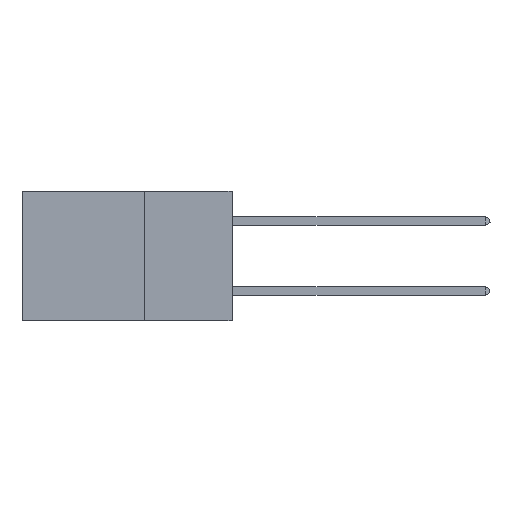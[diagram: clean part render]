
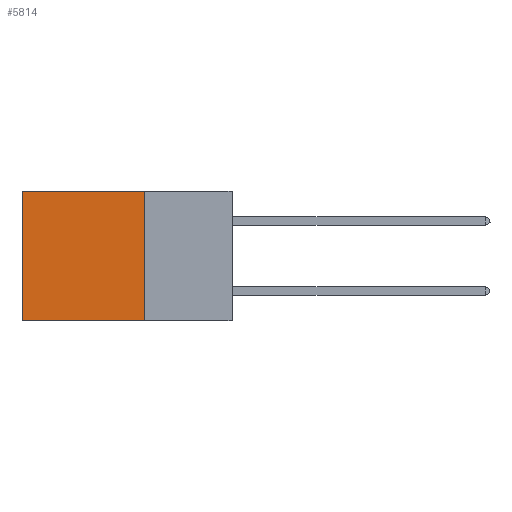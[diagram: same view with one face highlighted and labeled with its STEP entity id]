
A CAD part, left-side view. The second image highlights one B-rep face of the part: STEP entity #5814.
In plain terms, the highlighted planar face has unit normal (-1, 0, 0).
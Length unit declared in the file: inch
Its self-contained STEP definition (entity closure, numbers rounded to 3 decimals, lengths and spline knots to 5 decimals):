
#2529 = LINE ( 'NONE', #17342, #2656 ) ;
#2656 = VECTOR ( 'NONE', #24627, 39.37008 ) ;
#3174 = LINE ( 'NONE', #11003, #7167 ) ;
#3497 = DIRECTION ( 'NONE',  ( 0., 1., 0. ) ) ;
#5602 = VECTOR ( 'NONE', #5609, 39.37008 ) ;
#5607 = VERTEX_POINT ( 'NONE', #26257 ) ;
#5609 = DIRECTION ( 'NONE',  ( 0., 1., 0. ) ) ;
#5814 = ADVANCED_FACE ( 'NONE', ( #15115 ), #10674, .F. ) ;
#5888 = DIRECTION ( 'NONE',  ( 1., 0., 0. ) ) ;
#6472 = EDGE_CURVE ( 'NONE', #19785, #5607, #18094, .T. ) ;
#7167 = VECTOR ( 'NONE', #3497, 39.37008 ) ;
#10674 = PLANE ( 'NONE',  #23064 ) ;
#11003 = CARTESIAN_POINT ( 'NONE',  ( 0.2875, 0.25, 0. ) ) ;
#12568 = EDGE_LOOP ( 'NONE', ( #24395, #30051, #25993, #19257 ) ) ;
#13399 = VERTEX_POINT ( 'NONE', #23715 ) ;
#13793 = CARTESIAN_POINT ( 'NONE',  ( 0.2875, 0.25, 0. ) ) ;
#15115 = FACE_OUTER_BOUND ( 'NONE', #12568, .T. ) ;
#17342 = CARTESIAN_POINT ( 'NONE',  ( 0.2875, 0.6, 0. ) ) ;
#17708 = CARTESIAN_POINT ( 'NONE',  ( 0.2875, 0.25, -0.37 ) ) ;
#18094 = LINE ( 'NONE', #13793, #31265 ) ;
#19257 = ORIENTED_EDGE ( 'NONE', *, *, #26668, .T. ) ;
#19785 = VERTEX_POINT ( 'NONE', #27792 ) ;
#19858 = CARTESIAN_POINT ( 'NONE',  ( 0.2875, 0.25, 0. ) ) ;
#20336 = DIRECTION ( 'NONE',  ( 0., 0., -1. ) ) ;
#22622 = LINE ( 'NONE', #17708, #5602 ) ;
#23064 = AXIS2_PLACEMENT_3D ( 'NONE', #19858, #5888, #20336 ) ;
#23715 = CARTESIAN_POINT ( 'NONE',  ( 0.2875, 0.6, 0. ) ) ;
#24395 = ORIENTED_EDGE ( 'NONE', *, *, #31146, .T. ) ;
#24627 = DIRECTION ( 'NONE',  ( 0., 0., -1. ) ) ;
#25993 = ORIENTED_EDGE ( 'NONE', *, *, #6472, .F. ) ;
#26257 = CARTESIAN_POINT ( 'NONE',  ( 0.2875, 0.25, -0.37 ) ) ;
#26270 = EDGE_CURVE ( 'NONE', #5607, #27166, #22622, .T. ) ;
#26668 = EDGE_CURVE ( 'NONE', #19785, #13399, #3174, .T. ) ;
#27166 = VERTEX_POINT ( 'NONE', #30824 ) ;
#27782 = DIRECTION ( 'NONE',  ( 0., 0., -1. ) ) ;
#27792 = CARTESIAN_POINT ( 'NONE',  ( 0.2875, 0.25, 0. ) ) ;
#30051 = ORIENTED_EDGE ( 'NONE', *, *, #26270, .F. ) ;
#30824 = CARTESIAN_POINT ( 'NONE',  ( 0.2875, 0.6, -0.37 ) ) ;
#31146 = EDGE_CURVE ( 'NONE', #13399, #27166, #2529, .T. ) ;
#31265 = VECTOR ( 'NONE', #27782, 39.37008 ) ;
